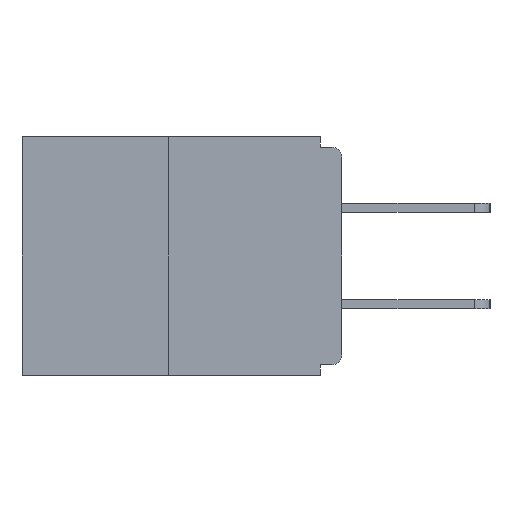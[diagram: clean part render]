
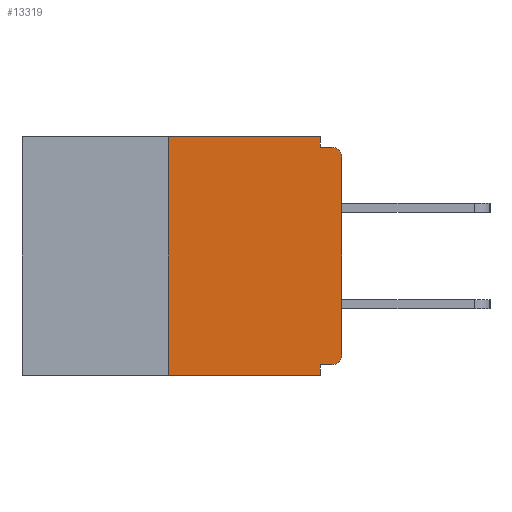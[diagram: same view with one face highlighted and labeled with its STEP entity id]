
A CAD part, left-side view. The second image highlights one B-rep face of the part: STEP entity #13319.
In plain terms, the highlighted planar face has unit normal (-1, 0, 0).
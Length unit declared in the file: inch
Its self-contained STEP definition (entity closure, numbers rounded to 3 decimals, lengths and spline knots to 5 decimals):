
#54 = EDGE_CURVE ( 'NONE', #6597, #3408, #4053, .T. ) ;
#129 = EDGE_LOOP ( 'NONE', ( #7753, #4254, #10254, #8671, #2368, #7152, #8650, #9169, #9636, #6678 ) ) ;
#198 = VERTEX_POINT ( 'NONE', #11983 ) ;
#244 = DIRECTION ( 'NONE',  ( 0., -1., 0. ) ) ;
#763 = CARTESIAN_POINT ( 'NONE',  ( 0., 0., 0. ) ) ;
#812 = DIRECTION ( 'NONE',  ( -1., 0., 0. ) ) ;
#1026 = CARTESIAN_POINT ( 'NONE',  ( 0., 0.25, 0. ) ) ;
#1044 = DIRECTION ( 'NONE',  ( 0., 1., 0. ) ) ;
#1161 = VECTOR ( 'NONE', #12273, 39.37008 ) ;
#1203 = DIRECTION ( 'NONE',  ( 0., 0., -1. ) ) ;
#1702 = LINE ( 'NONE', #13396, #1161 ) ;
#1796 = CIRCLE ( 'NONE', #2958, 0.015 ) ;
#1801 = CARTESIAN_POINT ( 'NONE',  ( 0., 0.015, -0.313 ) ) ;
#1901 = LINE ( 'NONE', #1026, #10127 ) ;
#2054 = EDGE_CURVE ( 'NONE', #13346, #11769, #11359, .T. ) ;
#2368 = ORIENTED_EDGE ( 'NONE', *, *, #11557, .F. ) ;
#2384 = EDGE_CURVE ( 'NONE', #4131, #4980, #3158, .T. ) ;
#2457 = LINE ( 'NONE', #6956, #14272 ) ;
#2632 = DIRECTION ( 'NONE',  ( 0., 0., -1. ) ) ;
#2958 = AXIS2_PLACEMENT_3D ( 'NONE', #1801, #812, #14554 ) ;
#3047 = DIRECTION ( 'NONE',  ( 0., 0., 1. ) ) ;
#3158 = LINE ( 'NONE', #8073, #13175 ) ;
#3237 = VERTEX_POINT ( 'NONE', #5802 ) ;
#3408 = VERTEX_POINT ( 'NONE', #4712 ) ;
#3726 = CIRCLE ( 'NONE', #7487, 0.015 ) ;
#3850 = VECTOR ( 'NONE', #1044, 39.37008 ) ;
#3947 = CARTESIAN_POINT ( 'NONE',  ( 0., 0., -0.313 ) ) ;
#4053 = LINE ( 'NONE', #763, #10878 ) ;
#4131 = VERTEX_POINT ( 'NONE', #11546 ) ;
#4254 = ORIENTED_EDGE ( 'NONE', *, *, #12298, .F. ) ;
#4712 = CARTESIAN_POINT ( 'NONE',  ( 0., 0., -0.03 ) ) ;
#4980 = VERTEX_POINT ( 'NONE', #13671 ) ;
#5584 = EDGE_CURVE ( 'NONE', #3408, #198, #3726, .T. ) ;
#5802 = CARTESIAN_POINT ( 'NONE',  ( 0., 0.015, -0.328 ) ) ;
#5815 = DIRECTION ( 'NONE',  ( 0., 0., -1. ) ) ;
#5945 = EDGE_CURVE ( 'NONE', #3237, #6597, #1796, .T. ) ;
#6046 = CARTESIAN_POINT ( 'NONE',  ( 0., 0.46, 0. ) ) ;
#6371 = FACE_OUTER_BOUND ( 'NONE', #129, .T. ) ;
#6597 = VERTEX_POINT ( 'NONE', #3947 ) ;
#6678 = ORIENTED_EDGE ( 'NONE', *, *, #11284, .F. ) ;
#6680 = VERTEX_POINT ( 'NONE', #9635 ) ;
#6956 = CARTESIAN_POINT ( 'NONE',  ( 0., 0.031, 0. ) ) ;
#7106 = LINE ( 'NONE', #10704, #9784 ) ;
#7152 = ORIENTED_EDGE ( 'NONE', *, *, #5945, .T. ) ;
#7159 = DIRECTION ( 'NONE',  ( 1., 0., 0. ) ) ;
#7487 = AXIS2_PLACEMENT_3D ( 'NONE', #14757, #7978, #5815 ) ;
#7529 = DIRECTION ( 'NONE',  ( 0., -1., 0. ) ) ;
#7753 = ORIENTED_EDGE ( 'NONE', *, *, #2054, .F. ) ;
#7978 = DIRECTION ( 'NONE',  ( -1., 0., 0. ) ) ;
#7981 = EDGE_CURVE ( 'NONE', #10700, #198, #7106, .T. ) ;
#8073 = CARTESIAN_POINT ( 'NONE',  ( 0., 0.46, -0.343 ) ) ;
#8340 = VECTOR ( 'NONE', #244, 39.37008 ) ;
#8650 = ORIENTED_EDGE ( 'NONE', *, *, #54, .T. ) ;
#8671 = ORIENTED_EDGE ( 'NONE', *, *, #12754, .F. ) ;
#9169 = ORIENTED_EDGE ( 'NONE', *, *, #5584, .T. ) ;
#9338 = AXIS2_PLACEMENT_3D ( 'NONE', #6046, #7159, #2632 ) ;
#9635 = CARTESIAN_POINT ( 'NONE',  ( 0., 0.031, -0.328 ) ) ;
#9636 = ORIENTED_EDGE ( 'NONE', *, *, #7981, .F. ) ;
#9784 = VECTOR ( 'NONE', #7529, 39.37008 ) ;
#10028 = DIRECTION ( 'NONE',  ( 0., 0., 1. ) ) ;
#10127 = VECTOR ( 'NONE', #10028, 39.37008 ) ;
#10254 = ORIENTED_EDGE ( 'NONE', *, *, #2384, .T. ) ;
#10326 = LINE ( 'NONE', #12249, #3850 ) ;
#10452 = DIRECTION ( 'NONE',  ( 0., -1., 0. ) ) ;
#10700 = VERTEX_POINT ( 'NONE', #11604 ) ;
#10704 = CARTESIAN_POINT ( 'NONE',  ( 0., 0., -0.015 ) ) ;
#10878 = VECTOR ( 'NONE', #3047, 39.37008 ) ;
#11284 = EDGE_CURVE ( 'NONE', #11769, #10700, #2457, .T. ) ;
#11343 = CARTESIAN_POINT ( 'NONE',  ( 0., 0.031, 0. ) ) ;
#11359 = LINE ( 'NONE', #12612, #8340 ) ;
#11546 = CARTESIAN_POINT ( 'NONE',  ( 0., 0.25, -0.343 ) ) ;
#11557 = EDGE_CURVE ( 'NONE', #3237, #6680, #10326, .T. ) ;
#11604 = CARTESIAN_POINT ( 'NONE',  ( 0., 0.031, -0.015 ) ) ;
#11769 = VERTEX_POINT ( 'NONE', #11343 ) ;
#11983 = CARTESIAN_POINT ( 'NONE',  ( 0., 0.015, -0.015 ) ) ;
#12136 = CARTESIAN_POINT ( 'NONE',  ( 0., 0.25, 0. ) ) ;
#12249 = CARTESIAN_POINT ( 'NONE',  ( 0., 0., -0.328 ) ) ;
#12273 = DIRECTION ( 'NONE',  ( 0., 0., -1. ) ) ;
#12298 = EDGE_CURVE ( 'NONE', #4131, #13346, #1901, .T. ) ;
#12612 = CARTESIAN_POINT ( 'NONE',  ( 0., 0.46, 0. ) ) ;
#12754 = EDGE_CURVE ( 'NONE', #6680, #4980, #1702, .T. ) ;
#12946 = PLANE ( 'NONE',  #9338 ) ;
#13175 = VECTOR ( 'NONE', #10452, 39.37008 ) ;
#13319 = ADVANCED_FACE ( 'NONE', ( #6371 ), #12946, .F. ) ;
#13346 = VERTEX_POINT ( 'NONE', #12136 ) ;
#13396 = CARTESIAN_POINT ( 'NONE',  ( 0., 0.031, -0.343 ) ) ;
#13671 = CARTESIAN_POINT ( 'NONE',  ( 0., 0.031, -0.343 ) ) ;
#14272 = VECTOR ( 'NONE', #1203, 39.37008 ) ;
#14554 = DIRECTION ( 'NONE',  ( 0., 0., -1. ) ) ;
#14757 = CARTESIAN_POINT ( 'NONE',  ( 0., 0.015, -0.03 ) ) ;
